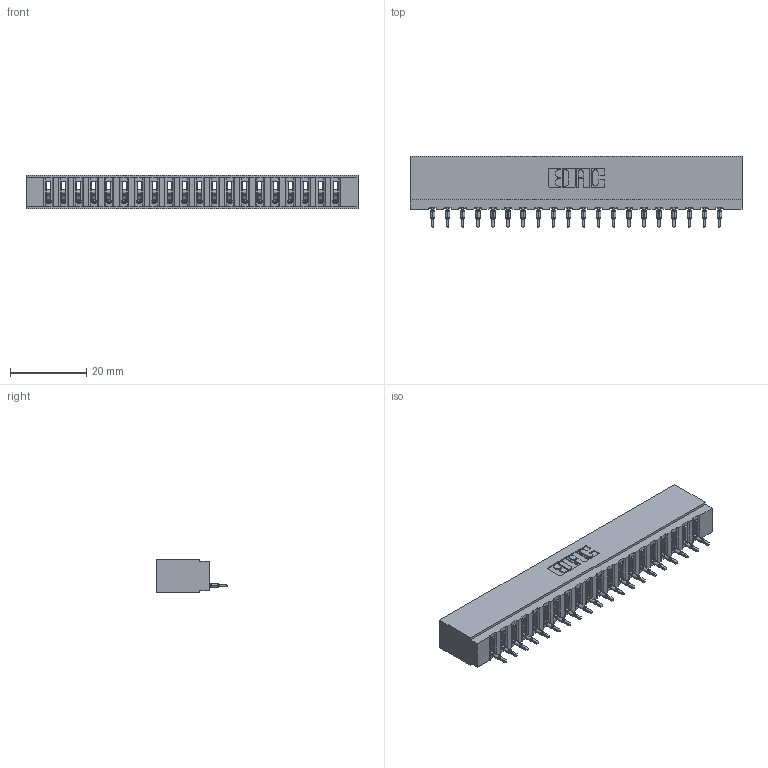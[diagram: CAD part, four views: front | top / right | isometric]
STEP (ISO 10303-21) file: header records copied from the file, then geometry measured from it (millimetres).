
FILE_DESCRIPTION (( 'STEP AP203' ), '1' );
FILE_NAME ('717-020-560-106.STEP', '2020-03-13T19:11:14', ( '' ), ( '' ), 'SwSTEP 2.0', 'SolidWorks 2016', '' );
FILE_SCHEMA (( 'CONFIG_CONTROL_DESIGN' ));
Length unit declared in the file: inch
Products named in the file (3): 745-292-001_560; 717-020-560-106; 717 Part_Insulator Option - 06
Assembly tree (21 placements, depth 2):
  717-020-560-106
    717 Part_Insulator Option - 06
    745-292-001_560  x20
Bounding box: 87.12 x 18.78 x 8.89 mm (x, y, z)
Volume: 7518 mm3; surface area: 10645.5 mm2
Topology: 21 solids, 21 shells, 2534 faces, 7051 edges, 4486 vertices
Faces by surface type: plane 1514, cylinder 500, bspline 400, torus 120
Entity records: 36954 total; most frequent: CARTESIAN_POINT 7015, ORIENTED_EDGE 6426, DIRECTION 5595, EDGE_CURVE 3213, LINE 2903, VECTOR 2903, VERTEX_POINT 2054, AXIS2_PLACEMENT_3D 1346
